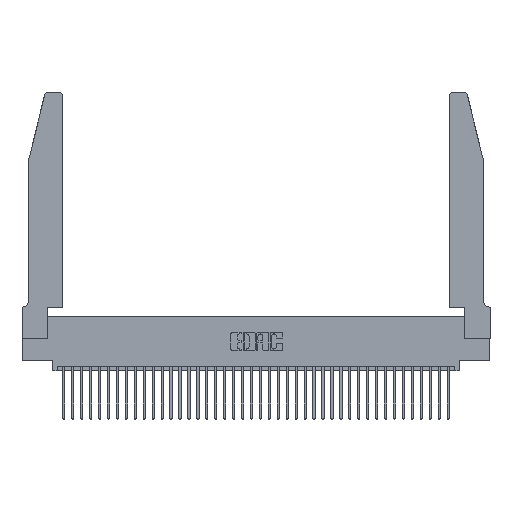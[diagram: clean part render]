
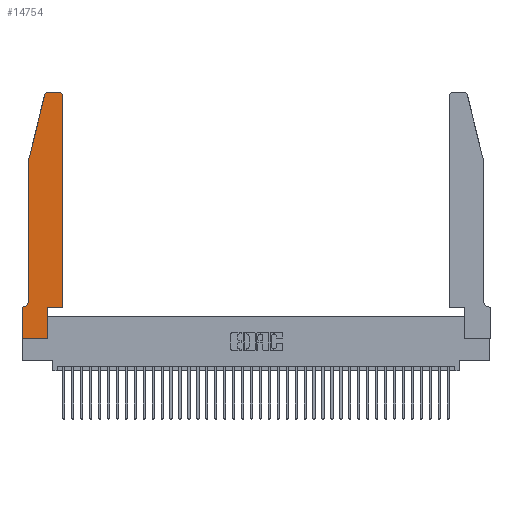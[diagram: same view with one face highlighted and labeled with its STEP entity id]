
A CAD part, top view. The second image highlights one B-rep face of the part: STEP entity #14754.
In plain terms, the highlighted planar face has unit normal (0, 0, 1).
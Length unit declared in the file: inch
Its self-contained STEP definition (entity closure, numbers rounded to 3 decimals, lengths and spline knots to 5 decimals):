
#79 = DIRECTION ( 'NONE',  ( 0., 0., 1. ) ) ;
#284 = AXIS2_PLACEMENT_3D ( 'NONE', #13160, #16053, #18969 ) ;
#901 = DIRECTION ( 'NONE',  ( 1., 0., 0. ) ) ;
#1064 = LINE ( 'NONE', #1538, #16228 ) ;
#1538 = CARTESIAN_POINT ( 'NONE',  ( 0.0755, 2., 0.37 ) ) ;
#4042 = ORIENTED_EDGE ( 'NONE', *, *, #22012, .T. ) ;
#4313 = FACE_OUTER_BOUND ( 'NONE', #32658, .T. ) ;
#4920 = VECTOR ( 'NONE', #13474, 39.37008 ) ;
#5346 = CARTESIAN_POINT ( 'NONE',  ( 0.4205, 2.75, 0.37 ) ) ;
#5414 = LINE ( 'NONE', #28913, #4920 ) ;
#6322 = EDGE_CURVE ( 'NONE', #21906, #32586, #7357, .T. ) ;
#7131 = CARTESIAN_POINT ( 'NONE',  ( 0., 0., 0.37 ) ) ;
#7146 = DIRECTION ( 'NONE',  ( 0., -1., 0. ) ) ;
#7274 = DIRECTION ( 'NONE',  ( 1., 0., 0. ) ) ;
#7333 = DIRECTION ( 'NONE',  ( 0., -1., 0. ) ) ;
#7357 = LINE ( 'NONE', #22436, #9235 ) ;
#7382 = VERTEX_POINT ( 'NONE', #24677 ) ;
#7857 = VERTEX_POINT ( 'NONE', #21998 ) ;
#8254 = ORIENTED_EDGE ( 'NONE', *, *, #25597, .T. ) ;
#8925 = VERTEX_POINT ( 'NONE', #35795 ) ;
#9235 = VECTOR ( 'NONE', #7333, 39.37008 ) ;
#9906 = PLANE ( 'NONE',  #15616 ) ;
#10005 = ORIENTED_EDGE ( 'NONE', *, *, #13968, .T. ) ;
#10753 = DIRECTION ( 'NONE',  ( -1., 0., 0. ) ) ;
#11369 = VECTOR ( 'NONE', #15204, 39.37008 ) ;
#11625 = CARTESIAN_POINT ( 'NONE',  ( 0.2865, 0.35, 0.37 ) ) ;
#12173 = ORIENTED_EDGE ( 'NONE', *, *, #27706, .T. ) ;
#12777 = LINE ( 'NONE', #28881, #30257 ) ;
#12863 = DIRECTION ( 'NONE',  ( 1., 0., 0. ) ) ;
#12984 = DIRECTION ( 'NONE',  ( 0., 0., 1. ) ) ;
#13154 = CARTESIAN_POINT ( 'NONE',  ( 0., 0., 0.37 ) ) ;
#13160 = CARTESIAN_POINT ( 'NONE',  ( 0.0055, 0.42, 0.37 ) ) ;
#13474 = DIRECTION ( 'NONE',  ( 0., 1., 0. ) ) ;
#13925 = VECTOR ( 'NONE', #14245, 39.37008 ) ;
#13968 = EDGE_CURVE ( 'NONE', #8925, #7857, #35157, .T. ) ;
#14092 = CARTESIAN_POINT ( 'NONE',  ( 0.4505, 2.72, 0.37 ) ) ;
#14245 = DIRECTION ( 'NONE',  ( 1., 0., 0. ) ) ;
#14754 = ADVANCED_FACE ( 'NONE', ( #4313 ), #9906, .T. ) ;
#14847 = LINE ( 'NONE', #7131, #36529 ) ;
#15204 = DIRECTION ( 'NONE',  ( 0., 1., 0. ) ) ;
#15616 = AXIS2_PLACEMENT_3D ( 'NONE', #24979, #12984, #901 ) ;
#15892 = CARTESIAN_POINT ( 'NONE',  ( 0.4205, 2.72, 0.37 ) ) ;
#16053 = DIRECTION ( 'NONE',  ( 0., 0., -1. ) ) ;
#16228 = VECTOR ( 'NONE', #24824, 39.37008 ) ;
#16584 = LINE ( 'NONE', #23660, #11369 ) ;
#16928 = ORIENTED_EDGE ( 'NONE', *, *, #37342, .T. ) ;
#16960 = CIRCLE ( 'NONE', #31341, 0.03 ) ;
#17123 = EDGE_CURVE ( 'NONE', #38194, #29126, #16960, .T. ) ;
#17298 = ORIENTED_EDGE ( 'NONE', *, *, #21276, .T. ) ;
#17511 = VERTEX_POINT ( 'NONE', #11625 ) ;
#18692 = CARTESIAN_POINT ( 'NONE',  ( 0.25487, 2.72718, 0.37 ) ) ;
#18969 = DIRECTION ( 'NONE',  ( -1., 0., 0. ) ) ;
#19450 = DIRECTION ( 'NONE',  ( 0., 0., 1. ) ) ;
#19577 = CARTESIAN_POINT ( 'NONE',  ( 0.4505, 0.35, 0.37 ) ) ;
#20134 = ORIENTED_EDGE ( 'NONE', *, *, #6322, .T. ) ;
#20909 = ORIENTED_EDGE ( 'NONE', *, *, #17123, .T. ) ;
#20950 = VERTEX_POINT ( 'NONE', #19577 ) ;
#21276 = EDGE_CURVE ( 'NONE', #25283, #17511, #16584, .T. ) ;
#21433 = EDGE_CURVE ( 'NONE', #22992, #29683, #31670, .T. ) ;
#21906 = VERTEX_POINT ( 'NONE', #27968 ) ;
#21998 = CARTESIAN_POINT ( 'NONE',  ( 0., 0., 0.37 ) ) ;
#22012 = EDGE_CURVE ( 'NONE', #32586, #7382, #36859, .T. ) ;
#22436 = CARTESIAN_POINT ( 'NONE',  ( 0.0755, 2., 0.37 ) ) ;
#22992 = VERTEX_POINT ( 'NONE', #32642 ) ;
#23660 = CARTESIAN_POINT ( 'NONE',  ( 0.2865, 0.35, 0.37 ) ) ;
#24462 = EDGE_CURVE ( 'NONE', #20950, #38194, #5414, .T. ) ;
#24677 = CARTESIAN_POINT ( 'NONE',  ( 0.0055, 0.35, 0.37 ) ) ;
#24824 = DIRECTION ( 'NONE',  ( -0.239, -0.971, 0. ) ) ;
#24878 = ORIENTED_EDGE ( 'NONE', *, *, #21433, .T. ) ;
#24979 = CARTESIAN_POINT ( 'NONE',  ( 0., 0.35, 0.37 ) ) ;
#25283 = VERTEX_POINT ( 'NONE', #27070 ) ;
#25597 = EDGE_CURVE ( 'NONE', #17511, #20950, #31361, .T. ) ;
#25673 = DIRECTION ( 'NONE',  ( 1., 0., 0. ) ) ;
#26125 = CARTESIAN_POINT ( 'NONE',  ( 0.0755, 0.42, 0.37 ) ) ;
#26144 = EDGE_CURVE ( 'NONE', #7857, #25283, #14847, .T. ) ;
#27070 = CARTESIAN_POINT ( 'NONE',  ( 0.2865, 0., 0.37 ) ) ;
#27117 = VECTOR ( 'NONE', #28900, 39.37008 ) ;
#27706 = EDGE_CURVE ( 'NONE', #29126, #22992, #12777, .T. ) ;
#27870 = CARTESIAN_POINT ( 'NONE',  ( 0.284, 2.72, 0.37 ) ) ;
#27968 = CARTESIAN_POINT ( 'NONE',  ( 0.0755, 2., 0.37 ) ) ;
#28881 = CARTESIAN_POINT ( 'NONE',  ( 0.2605, 2.75, 0.37 ) ) ;
#28900 = DIRECTION ( 'NONE',  ( -1., 0., 0. ) ) ;
#28913 = CARTESIAN_POINT ( 'NONE',  ( 0.4505, 0.35, 0.37 ) ) ;
#29126 = VERTEX_POINT ( 'NONE', #5346 ) ;
#29683 = VERTEX_POINT ( 'NONE', #18692 ) ;
#30257 = VECTOR ( 'NONE', #10753, 39.37008 ) ;
#30726 = EDGE_CURVE ( 'NONE', #7382, #8925, #38427, .T. ) ;
#31208 = ORIENTED_EDGE ( 'NONE', *, *, #24462, .T. ) ;
#31341 = AXIS2_PLACEMENT_3D ( 'NONE', #15892, #19450, #12863 ) ;
#31361 = LINE ( 'NONE', #32190, #13925 ) ;
#31670 = CIRCLE ( 'NONE', #35513, 0.03 ) ;
#32190 = CARTESIAN_POINT ( 'NONE',  ( 0.4505, 0.35, 0.37 ) ) ;
#32586 = VERTEX_POINT ( 'NONE', #26125 ) ;
#32628 = CARTESIAN_POINT ( 'NONE',  ( 0.0755, 0.35, 0.37 ) ) ;
#32642 = CARTESIAN_POINT ( 'NONE',  ( 0.284, 2.75, 0.37 ) ) ;
#32658 = EDGE_LOOP ( 'NONE', ( #12173, #24878, #16928, #20134, #4042, #33527, #10005, #35427, #17298, #8254, #31208, #20909 ) ) ;
#32813 = VECTOR ( 'NONE', #7146, 39.37008 ) ;
#33527 = ORIENTED_EDGE ( 'NONE', *, *, #30726, .T. ) ;
#35157 = LINE ( 'NONE', #13154, #32813 ) ;
#35427 = ORIENTED_EDGE ( 'NONE', *, *, #26144, .T. ) ;
#35513 = AXIS2_PLACEMENT_3D ( 'NONE', #27870, #79, #7274 ) ;
#35795 = CARTESIAN_POINT ( 'NONE',  ( 0., 0.35, 0.37 ) ) ;
#36529 = VECTOR ( 'NONE', #25673, 39.37008 ) ;
#36859 = CIRCLE ( 'NONE', #284, 0.07 ) ;
#37342 = EDGE_CURVE ( 'NONE', #29683, #21906, #1064, .T. ) ;
#38194 = VERTEX_POINT ( 'NONE', #14092 ) ;
#38427 = LINE ( 'NONE', #32628, #27117 ) ;
